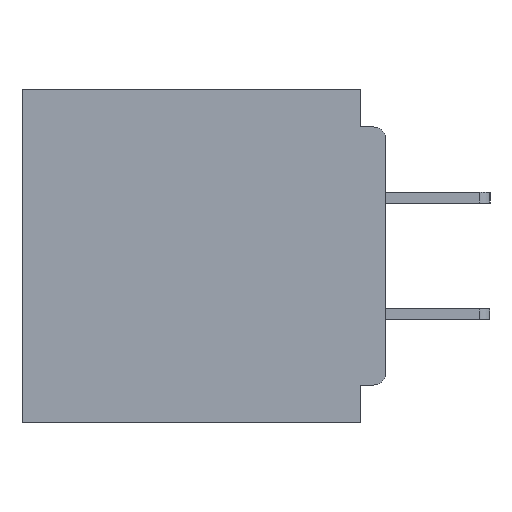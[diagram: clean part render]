
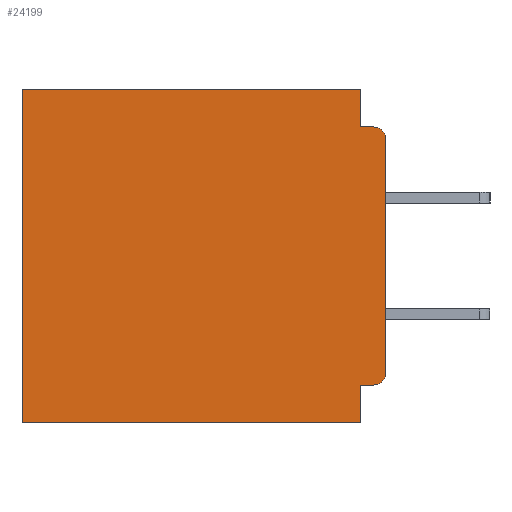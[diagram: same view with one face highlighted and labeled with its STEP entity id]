
A CAD part, left-side view. The second image highlights one B-rep face of the part: STEP entity #24199.
In plain terms, the highlighted planar face has unit normal (-1, 0, 0).
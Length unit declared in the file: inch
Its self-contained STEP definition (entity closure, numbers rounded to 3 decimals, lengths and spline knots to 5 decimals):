
#1499 = ORIENTED_EDGE ( 'NONE', *, *, #40371, .F. ) ;
#1860 = LINE ( 'NONE', #30363, #39003 ) ;
#1956 = CARTESIAN_POINT ( 'NONE',  ( 0.3, 0.015, -0.06 ) ) ;
#2041 = EDGE_CURVE ( 'NONE', #27151, #38826, #2720, .T. ) ;
#2720 = LINE ( 'NONE', #35307, #26003 ) ;
#3705 = CARTESIAN_POINT ( 'NONE',  ( 0.3, 0., -0.045 ) ) ;
#3832 = ORIENTED_EDGE ( 'NONE', *, *, #19306, .T. ) ;
#4454 = EDGE_CURVE ( 'NONE', #6920, #6103, #37133, .T. ) ;
#4933 = EDGE_CURVE ( 'NONE', #24678, #38826, #24819, .T. ) ;
#4991 = EDGE_CURVE ( 'NONE', #33493, #5792, #14408, .T. ) ;
#5119 = DIRECTION ( 'NONE',  ( 0., 0., -1. ) ) ;
#5369 = CARTESIAN_POINT ( 'NONE',  ( 0.3, 0.015, -0.045 ) ) ;
#5792 = VERTEX_POINT ( 'NONE', #5369 ) ;
#6103 = VERTEX_POINT ( 'NONE', #18063 ) ;
#6240 = AXIS2_PLACEMENT_3D ( 'NONE', #10099, #35326, #16466 ) ;
#6393 = EDGE_CURVE ( 'NONE', #10988, #24678, #36526, .T. ) ;
#6506 = ORIENTED_EDGE ( 'NONE', *, *, #20591, .F. ) ;
#6920 = VERTEX_POINT ( 'NONE', #34236 ) ;
#6923 = AXIS2_PLACEMENT_3D ( 'NONE', #1956, #24095, #5119 ) ;
#7054 = EDGE_CURVE ( 'NONE', #10988, #33493, #10831, .T. ) ;
#7300 = AXIS2_PLACEMENT_3D ( 'NONE', #27142, #33353, #14429 ) ;
#7888 = CARTESIAN_POINT ( 'NONE',  ( 0.3, 0.437, -0.4 ) ) ;
#9267 = VECTOR ( 'NONE', #39854, 39.37008 ) ;
#10099 = CARTESIAN_POINT ( 'NONE',  ( 0.3, 0., -0.4 ) ) ;
#10163 = FACE_OUTER_BOUND ( 'NONE', #17685, .T. ) ;
#10382 = CARTESIAN_POINT ( 'NONE',  ( 0.3, 0.031, 0. ) ) ;
#10831 = LINE ( 'NONE', #10382, #26663 ) ;
#10988 = VERTEX_POINT ( 'NONE', #33911 ) ;
#11334 = DIRECTION ( 'NONE',  ( 0., 0., -1. ) ) ;
#11573 = CARTESIAN_POINT ( 'NONE',  ( 0.3, 0., -0.355 ) ) ;
#14408 = LINE ( 'NONE', #3705, #38530 ) ;
#14429 = DIRECTION ( 'NONE',  ( 0., 0., -1. ) ) ;
#14565 = DIRECTION ( 'NONE',  ( 0., 0., -1. ) ) ;
#14909 = DIRECTION ( 'NONE',  ( 0., 1., 0. ) ) ;
#15165 = DIRECTION ( 'NONE',  ( 0., 0., -1. ) ) ;
#15526 = CARTESIAN_POINT ( 'NONE',  ( 0.3, 0.031, -0.4 ) ) ;
#16399 = VERTEX_POINT ( 'NONE', #28851 ) ;
#16406 = VECTOR ( 'NONE', #11334, 39.37008 ) ;
#16466 = DIRECTION ( 'NONE',  ( 0., 0., -1. ) ) ;
#16864 = ORIENTED_EDGE ( 'NONE', *, *, #2041, .F. ) ;
#17685 = EDGE_LOOP ( 'NONE', ( #34472, #3832, #24789, #17691, #22805, #22718, #16864, #6506, #1499, #33111 ) ) ;
#17691 = ORIENTED_EDGE ( 'NONE', *, *, #7054, .F. ) ;
#17800 = VECTOR ( 'NONE', #29138, 39.37008 ) ;
#17868 = CARTESIAN_POINT ( 'NONE',  ( 0.3, 0., -0.4 ) ) ;
#18063 = CARTESIAN_POINT ( 'NONE',  ( 0.3, 0., -0.34 ) ) ;
#18489 = CARTESIAN_POINT ( 'NONE',  ( 0.3, 0.031, -0.045 ) ) ;
#18539 = LINE ( 'NONE', #11573, #27985 ) ;
#19306 = EDGE_CURVE ( 'NONE', #19513, #5792, #20423, .T. ) ;
#19513 = VERTEX_POINT ( 'NONE', #40649 ) ;
#20423 = CIRCLE ( 'NONE', #6923, 0.015 ) ;
#20591 = EDGE_CURVE ( 'NONE', #16399, #27151, #1860, .T. ) ;
#22694 = PLANE ( 'NONE',  #6240 ) ;
#22718 = ORIENTED_EDGE ( 'NONE', *, *, #4933, .T. ) ;
#22805 = ORIENTED_EDGE ( 'NONE', *, *, #6393, .T. ) ;
#24095 = DIRECTION ( 'NONE',  ( -1., 0., 0. ) ) ;
#24199 = ADVANCED_FACE ( 'NONE', ( #10163 ), #22694, .F. ) ;
#24365 = CARTESIAN_POINT ( 'NONE',  ( 0.3, 0.437, -0.4 ) ) ;
#24678 = VERTEX_POINT ( 'NONE', #28156 ) ;
#24789 = ORIENTED_EDGE ( 'NONE', *, *, #4991, .F. ) ;
#24819 = LINE ( 'NONE', #24365, #16406 ) ;
#26003 = VECTOR ( 'NONE', #14909, 39.37008 ) ;
#26663 = VECTOR ( 'NONE', #15165, 39.37008 ) ;
#27142 = CARTESIAN_POINT ( 'NONE',  ( 0.3, 0.015, -0.34 ) ) ;
#27151 = VERTEX_POINT ( 'NONE', #15526 ) ;
#27985 = VECTOR ( 'NONE', #33650, 39.37008 ) ;
#28156 = CARTESIAN_POINT ( 'NONE',  ( 0.3, 0.437, 0. ) ) ;
#28785 = DIRECTION ( 'NONE',  ( 0., -1., 0. ) ) ;
#28851 = CARTESIAN_POINT ( 'NONE',  ( 0.3, 0.031, -0.355 ) ) ;
#29138 = DIRECTION ( 'NONE',  ( 0., 1., 0. ) ) ;
#29144 = CARTESIAN_POINT ( 'NONE',  ( 0.3, 0., 0. ) ) ;
#30363 = CARTESIAN_POINT ( 'NONE',  ( 0.3, 0.031, -0.4 ) ) ;
#33111 = ORIENTED_EDGE ( 'NONE', *, *, #4454, .T. ) ;
#33353 = DIRECTION ( 'NONE',  ( -1., 0., 0. ) ) ;
#33483 = LINE ( 'NONE', #17868, #9267 ) ;
#33493 = VERTEX_POINT ( 'NONE', #18489 ) ;
#33650 = DIRECTION ( 'NONE',  ( 0., 1., 0. ) ) ;
#33911 = CARTESIAN_POINT ( 'NONE',  ( 0.3, 0.031, 0. ) ) ;
#34236 = CARTESIAN_POINT ( 'NONE',  ( 0.3, 0.015, -0.355 ) ) ;
#34472 = ORIENTED_EDGE ( 'NONE', *, *, #34643, .F. ) ;
#34643 = EDGE_CURVE ( 'NONE', #19513, #6103, #33483, .T. ) ;
#35307 = CARTESIAN_POINT ( 'NONE',  ( 0.3, 0., -0.4 ) ) ;
#35326 = DIRECTION ( 'NONE',  ( 1., 0., 0. ) ) ;
#36526 = LINE ( 'NONE', #29144, #17800 ) ;
#37133 = CIRCLE ( 'NONE', #7300, 0.015 ) ;
#38530 = VECTOR ( 'NONE', #28785, 39.37008 ) ;
#38826 = VERTEX_POINT ( 'NONE', #7888 ) ;
#39003 = VECTOR ( 'NONE', #14565, 39.37008 ) ;
#39854 = DIRECTION ( 'NONE',  ( 0., 0., -1. ) ) ;
#40371 = EDGE_CURVE ( 'NONE', #6920, #16399, #18539, .T. ) ;
#40649 = CARTESIAN_POINT ( 'NONE',  ( 0.3, 0., -0.06 ) ) ;
